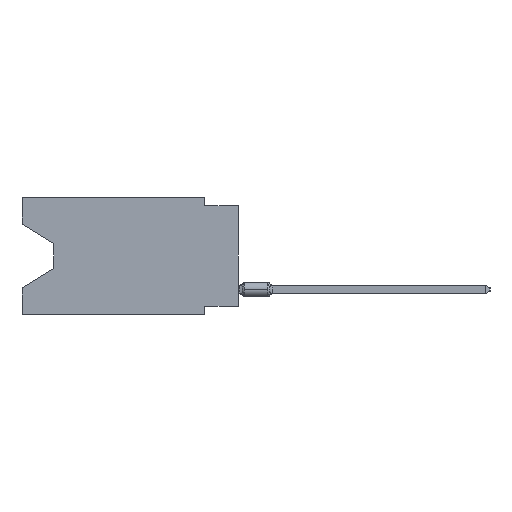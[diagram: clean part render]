
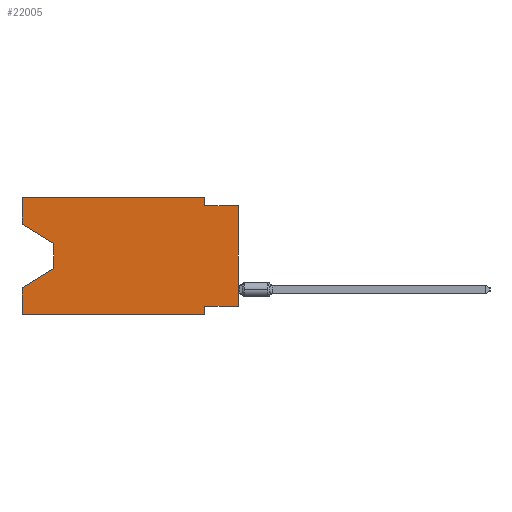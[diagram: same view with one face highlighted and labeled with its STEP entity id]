
A CAD part, left-side view. The second image highlights one B-rep face of the part: STEP entity #22005.
In plain terms, the highlighted planar face has unit normal (-1, 0, 0).
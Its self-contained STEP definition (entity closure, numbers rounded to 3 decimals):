
#1482 = VECTOR ( 'NONE', #39657, 1000. ) ;
#1600 = VECTOR ( 'NONE', #47385, 1000. ) ;
#1910 = EDGE_CURVE ( 'NONE', #45011, #10272, #7033, .T. ) ;
#2577 = VECTOR ( 'NONE', #11433, 1000. ) ;
#2927 = VERTEX_POINT ( 'NONE', #26104 ) ;
#3438 = ORIENTED_EDGE ( 'NONE', *, *, #40810, .F. ) ;
#3774 = CARTESIAN_POINT ( 'NONE',  ( 0., 16.383, 0. ) ) ;
#3799 = CARTESIAN_POINT ( 'NONE',  ( 0., 13.97, -5.385 ) ) ;
#3980 = CARTESIAN_POINT ( 'NONE',  ( 0., 2.54, -0.635 ) ) ;
#4671 = EDGE_CURVE ( 'NONE', #21261, #45011, #20349, .T. ) ;
#5527 = VERTEX_POINT ( 'NONE', #33263 ) ;
#6888 = EDGE_CURVE ( 'NONE', #19877, #38714, #8385, .T. ) ;
#7033 = LINE ( 'NONE', #21101, #24756 ) ;
#7371 = VECTOR ( 'NONE', #45872, 1000. ) ;
#7461 = ORIENTED_EDGE ( 'NONE', *, *, #6888, .T. ) ;
#7961 = VERTEX_POINT ( 'NONE', #34229 ) ;
#8385 = LINE ( 'NONE', #3799, #1482 ) ;
#8674 = LINE ( 'NONE', #43439, #35857 ) ;
#8783 = CARTESIAN_POINT ( 'NONE',  ( 0., 0., -0.635 ) ) ;
#8966 = ORIENTED_EDGE ( 'NONE', *, *, #40830, .T. ) ;
#10272 = VERTEX_POINT ( 'NONE', #8783 ) ;
#10331 = CARTESIAN_POINT ( 'NONE',  ( 0., 16.383, -6.852 ) ) ;
#10805 = EDGE_CURVE ( 'NONE', #2927, #38714, #31411, .T. ) ;
#11433 = DIRECTION ( 'NONE',  ( 0., -1., 0. ) ) ;
#11655 = CARTESIAN_POINT ( 'NONE',  ( 0., 16.383, -8.89 ) ) ;
#11950 = DIRECTION ( 'NONE',  ( 0., -1., 0. ) ) ;
#12208 = AXIS2_PLACEMENT_3D ( 'NONE', #3774, #21286, #38786 ) ;
#14355 = VECTOR ( 'NONE', #37521, 1000. ) ;
#15259 = VECTOR ( 'NONE', #30830, 1000. ) ;
#16687 = DIRECTION ( 'NONE',  ( 0., 0., 1. ) ) ;
#17573 = ORIENTED_EDGE ( 'NONE', *, *, #1910, .F. ) ;
#19061 = VECTOR ( 'NONE', #56031, 1000. ) ;
#19646 = ORIENTED_EDGE ( 'NONE', *, *, #54867, .T. ) ;
#19877 = VERTEX_POINT ( 'NONE', #39059 ) ;
#20290 = LINE ( 'NONE', #28633, #14355 ) ;
#20349 = LINE ( 'NONE', #54543, #41177 ) ;
#21101 = CARTESIAN_POINT ( 'NONE',  ( 0., 0., -0.635 ) ) ;
#21261 = VERTEX_POINT ( 'NONE', #30400 ) ;
#21286 = DIRECTION ( 'NONE',  ( 1., 0., 0. ) ) ;
#22005 = ADVANCED_FACE ( 'NONE', ( #47134 ), #43123, .F. ) ;
#22387 = VERTEX_POINT ( 'NONE', #29833 ) ;
#23746 = LINE ( 'NONE', #45570, #7371 ) ;
#24522 = VERTEX_POINT ( 'NONE', #26284 ) ;
#24756 = VECTOR ( 'NONE', #38018, 1000. ) ;
#25426 = ORIENTED_EDGE ( 'NONE', *, *, #35582, .F. ) ;
#25579 = LINE ( 'NONE', #51468, #34006 ) ;
#26104 = CARTESIAN_POINT ( 'NONE',  ( 0., 16.383, -8.89 ) ) ;
#26284 = CARTESIAN_POINT ( 'NONE',  ( 0., 0., -8.255 ) ) ;
#27555 = VERTEX_POINT ( 'NONE', #39108 ) ;
#28546 = ORIENTED_EDGE ( 'NONE', *, *, #55552, .F. ) ;
#28633 = CARTESIAN_POINT ( 'NONE',  ( 0., 0., 0. ) ) ;
#29833 = CARTESIAN_POINT ( 'NONE',  ( 0., 13.97, -3.505 ) ) ;
#29872 = LINE ( 'NONE', #56571, #1600 ) ;
#30400 = CARTESIAN_POINT ( 'NONE',  ( 0., 2.54, 0. ) ) ;
#30830 = DIRECTION ( 'NONE',  ( 0., 0., 1. ) ) ;
#31411 = LINE ( 'NONE', #48657, #15259 ) ;
#32502 = EDGE_CURVE ( 'NONE', #27555, #21261, #55384, .T. ) ;
#33263 = CARTESIAN_POINT ( 'NONE',  ( 0., 16.383, -2.038 ) ) ;
#34006 = VECTOR ( 'NONE', #16687, 1000. ) ;
#34127 = CARTESIAN_POINT ( 'NONE',  ( 0., 2.54, -8.255 ) ) ;
#34229 = CARTESIAN_POINT ( 'NONE',  ( 0., 2.54, -8.89 ) ) ;
#34834 = DIRECTION ( 'NONE',  ( 0., 0., -1. ) ) ;
#35582 = EDGE_CURVE ( 'NONE', #5527, #27555, #25579, .T. ) ;
#35857 = VECTOR ( 'NONE', #34834, 1000. ) ;
#36199 = VECTOR ( 'NONE', #11950, 1000. ) ;
#37244 = ORIENTED_EDGE ( 'NONE', *, *, #32502, .F. ) ;
#37521 = DIRECTION ( 'NONE',  ( 0., 0., 1. ) ) ;
#37582 = EDGE_CURVE ( 'NONE', #2927, #7961, #46707, .T. ) ;
#37847 = DIRECTION ( 'NONE',  ( 0., 0., -1. ) ) ;
#38018 = DIRECTION ( 'NONE',  ( 0., -1., 0. ) ) ;
#38714 = VERTEX_POINT ( 'NONE', #10331 ) ;
#38786 = DIRECTION ( 'NONE',  ( 0., 0., -1. ) ) ;
#39059 = CARTESIAN_POINT ( 'NONE',  ( 0., 13.97, -5.385 ) ) ;
#39108 = CARTESIAN_POINT ( 'NONE',  ( 0., 16.383, 0. ) ) ;
#39374 = EDGE_CURVE ( 'NONE', #24522, #10272, #20290, .T. ) ;
#39657 = DIRECTION ( 'NONE',  ( 0., 0.855, -0.519 ) ) ;
#40810 = EDGE_CURVE ( 'NONE', #24522, #54632, #48232, .T. ) ;
#40830 = EDGE_CURVE ( 'NONE', #22387, #19877, #29872, .T. ) ;
#41074 = ORIENTED_EDGE ( 'NONE', *, *, #10805, .F. ) ;
#41177 = VECTOR ( 'NONE', #37847, 1000. ) ;
#43123 = PLANE ( 'NONE',  #12208 ) ;
#43370 = CARTESIAN_POINT ( 'NONE',  ( 0., 0., -8.255 ) ) ;
#43439 = CARTESIAN_POINT ( 'NONE',  ( 0., 2.54, -8.89 ) ) ;
#44545 = ORIENTED_EDGE ( 'NONE', *, *, #4671, .F. ) ;
#45011 = VERTEX_POINT ( 'NONE', #3980 ) ;
#45224 = EDGE_LOOP ( 'NONE', ( #19646, #8966, #7461, #41074, #48019, #28546, #3438, #47991, #17573, #44545, #37244, #25426 ) ) ;
#45570 = CARTESIAN_POINT ( 'NONE',  ( 0., 16.383, -2.038 ) ) ;
#45872 = DIRECTION ( 'NONE',  ( 0., -0.855, -0.519 ) ) ;
#46707 = LINE ( 'NONE', #11655, #36199 ) ;
#47134 = FACE_OUTER_BOUND ( 'NONE', #45224, .T. ) ;
#47385 = DIRECTION ( 'NONE',  ( 0., 0., -1. ) ) ;
#47991 = ORIENTED_EDGE ( 'NONE', *, *, #39374, .T. ) ;
#48019 = ORIENTED_EDGE ( 'NONE', *, *, #37582, .T. ) ;
#48232 = LINE ( 'NONE', #43370, #19061 ) ;
#48657 = CARTESIAN_POINT ( 'NONE',  ( 0., 16.383, 0. ) ) ;
#50802 = CARTESIAN_POINT ( 'NONE',  ( 0., 16.383, 0. ) ) ;
#51468 = CARTESIAN_POINT ( 'NONE',  ( 0., 16.383, 0. ) ) ;
#54543 = CARTESIAN_POINT ( 'NONE',  ( 0., 2.54, 0. ) ) ;
#54632 = VERTEX_POINT ( 'NONE', #34127 ) ;
#54867 = EDGE_CURVE ( 'NONE', #5527, #22387, #23746, .T. ) ;
#55384 = LINE ( 'NONE', #50802, #2577 ) ;
#55552 = EDGE_CURVE ( 'NONE', #54632, #7961, #8674, .T. ) ;
#56031 = DIRECTION ( 'NONE',  ( 0., 1., 0. ) ) ;
#56571 = CARTESIAN_POINT ( 'NONE',  ( 0., 13.97, -3.505 ) ) ;
